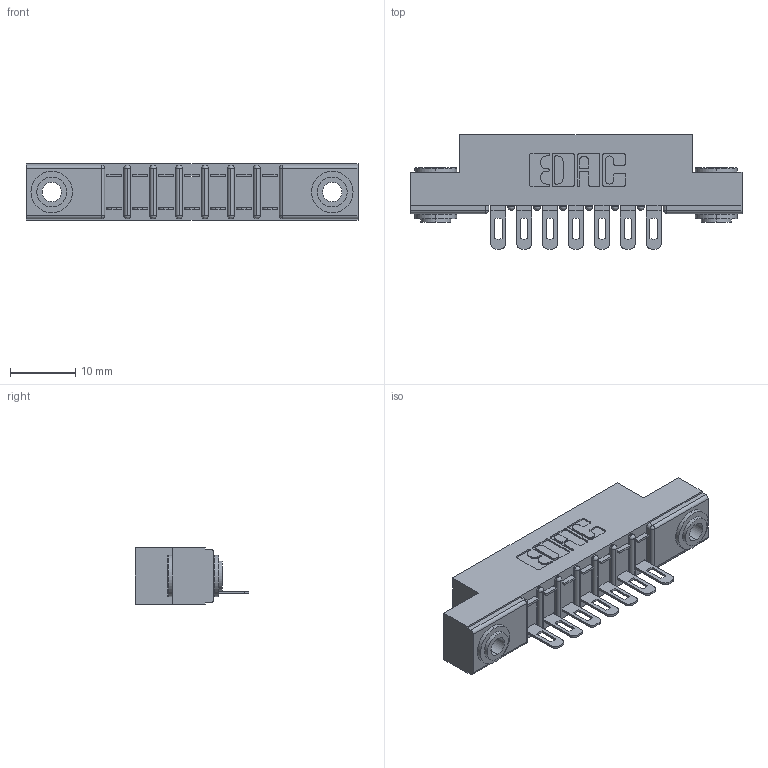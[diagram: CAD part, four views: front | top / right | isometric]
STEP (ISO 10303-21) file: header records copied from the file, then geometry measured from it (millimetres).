
FILE_DESCRIPTION (( 'STEP AP203' ), '1' );
FILE_NAME ('357-007-501-103.STEP', '2019-09-16T17:14:43', ( '' ), ( '' ), 'SwSTEP 2.0', 'SolidWorks 2016', '' );
FILE_SCHEMA (( 'CONFIG_CONTROL_DESIGN' ));
Length unit declared in the file: inch
Products named in the file (4): 357-007-501-103; 307 Part_.156 Dia Mounting Holes; 307-290-002_501; 345-250-002_345-250-002-102
Assembly tree (10 placements, depth 2):
  357-007-501-103
    307 Part_.156 Dia Mounting Holes
    307-290-002_501  x7
    345-250-002_345-250-002-102  x2
Bounding box: 50.75 x 17.42 x 8.71 mm (x, y, z)
Volume: 3349.9 mm3; surface area: 5549.9 mm2
Topology: 10 solids, 10 shells, 710 faces, 2101 edges, 1374 vertices
Faces by surface type: plane 402, cylinder 284, sphere 16, cone 8
Entity records: 12175 total; most frequent: CARTESIAN_POINT 2025, ORIENTED_EDGE 2006, DIRECTION 2003, EDGE_CURVE 1003, VECTOR 739, LINE 739, VERTEX_POINT 654, AXIS2_PLACEMENT_3D 632
